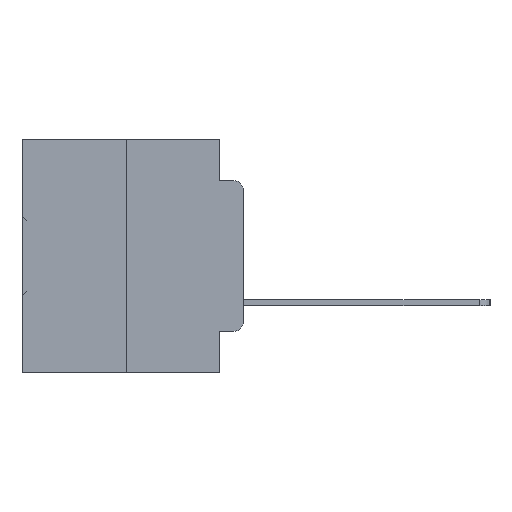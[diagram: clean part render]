
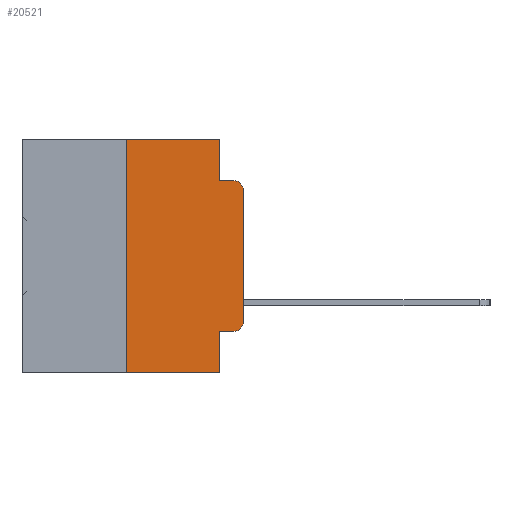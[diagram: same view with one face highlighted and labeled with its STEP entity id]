
A CAD part, left-side view. The second image highlights one B-rep face of the part: STEP entity #20521.
In plain terms, the highlighted planar face has unit normal (-1, 0, 0).
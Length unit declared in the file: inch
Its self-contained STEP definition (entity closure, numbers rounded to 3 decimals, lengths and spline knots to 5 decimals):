
#121 = LINE ( 'NONE', #28309, #34793 ) ;
#863 = DIRECTION ( 'NONE',  ( 0., -1., 0. ) ) ;
#1040 = CARTESIAN_POINT ( 'NONE',  ( 0., 0.25, 0. ) ) ;
#1068 = EDGE_CURVE ( 'NONE', #30678, #3644, #24633, .T. ) ;
#1377 = LINE ( 'NONE', #2020, #29755 ) ;
#2020 = CARTESIAN_POINT ( 'NONE',  ( 0., 0., 0. ) ) ;
#2580 = DIRECTION ( 'NONE',  ( 0., 0., -1. ) ) ;
#2614 = ORIENTED_EDGE ( 'NONE', *, *, #24018, .T. ) ;
#3579 = EDGE_LOOP ( 'NONE', ( #2614, #17501, #33373, #5268, #35038, #14469, #24235, #17936, #12300, #13171 ) ) ;
#3644 = VERTEX_POINT ( 'NONE', #8890 ) ;
#4977 = VERTEX_POINT ( 'NONE', #33874 ) ;
#5185 = AXIS2_PLACEMENT_3D ( 'NONE', #15831, #15921, #26658 ) ;
#5268 = ORIENTED_EDGE ( 'NONE', *, *, #10528, .F. ) ;
#6184 = VECTOR ( 'NONE', #16336, 39.37008 ) ;
#6233 = VECTOR ( 'NONE', #27719, 39.37008 ) ;
#6296 = CARTESIAN_POINT ( 'NONE',  ( 0., 0.051, -0.5 ) ) ;
#6386 = VERTEX_POINT ( 'NONE', #21506 ) ;
#6576 = CARTESIAN_POINT ( 'NONE',  ( 0., 0.051, -0.0885 ) ) ;
#6623 = LINE ( 'NONE', #24682, #20484 ) ;
#8890 = CARTESIAN_POINT ( 'NONE',  ( 0., 0.02, -0.0885 ) ) ;
#10528 = EDGE_CURVE ( 'NONE', #23998, #34937, #26033, .T. ) ;
#11148 = CARTESIAN_POINT ( 'NONE',  ( 0., 0.051, -0.0885 ) ) ;
#11433 = VERTEX_POINT ( 'NONE', #6296 ) ;
#11671 = EDGE_CURVE ( 'NONE', #6386, #18275, #14549, .T. ) ;
#12300 = ORIENTED_EDGE ( 'NONE', *, *, #12589, .T. ) ;
#12589 = EDGE_CURVE ( 'NONE', #4977, #23850, #22583, .T. ) ;
#12897 = CARTESIAN_POINT ( 'NONE',  ( 0., 0.02, -0.3915 ) ) ;
#13171 = ORIENTED_EDGE ( 'NONE', *, *, #20290, .T. ) ;
#13213 = CARTESIAN_POINT ( 'NONE',  ( 0., 0.051, 0. ) ) ;
#13529 = CARTESIAN_POINT ( 'NONE',  ( 0., 0.051, -0.4115 ) ) ;
#13761 = PLANE ( 'NONE',  #28790 ) ;
#14206 = VECTOR ( 'NONE', #863, 39.37008 ) ;
#14469 = ORIENTED_EDGE ( 'NONE', *, *, #11671, .F. ) ;
#14549 = LINE ( 'NONE', #1040, #35109 ) ;
#14850 = DIRECTION ( 'NONE',  ( 0., 0., -1. ) ) ;
#15708 = DIRECTION ( 'NONE',  ( 0., 0., -1. ) ) ;
#15831 = CARTESIAN_POINT ( 'NONE',  ( 0., 0.02, -0.1085 ) ) ;
#15921 = DIRECTION ( 'NONE',  ( -1., 0., 0. ) ) ;
#16018 = DIRECTION ( 'NONE',  ( 0., 0., -1. ) ) ;
#16134 = EDGE_CURVE ( 'NONE', #34937, #3644, #28594, .T. ) ;
#16336 = DIRECTION ( 'NONE',  ( 0., -1., 0. ) ) ;
#17501 = ORIENTED_EDGE ( 'NONE', *, *, #1068, .T. ) ;
#17936 = ORIENTED_EDGE ( 'NONE', *, *, #33659, .F. ) ;
#18275 = VERTEX_POINT ( 'NONE', #27821 ) ;
#18853 = FACE_OUTER_BOUND ( 'NONE', #3579, .T. ) ;
#19296 = DIRECTION ( 'NONE',  ( 1., 0., 0. ) ) ;
#20290 = EDGE_CURVE ( 'NONE', #23850, #25393, #32629, .T. ) ;
#20484 = VECTOR ( 'NONE', #27399, 39.37008 ) ;
#20521 = ADVANCED_FACE ( 'NONE', ( #18853 ), #13761, .F. ) ;
#20655 = EDGE_CURVE ( 'NONE', #6386, #11433, #20956, .T. ) ;
#20956 = LINE ( 'NONE', #22330, #6233 ) ;
#21506 = CARTESIAN_POINT ( 'NONE',  ( 0., 0.25, -0.5 ) ) ;
#21876 = CARTESIAN_POINT ( 'NONE',  ( 0., 0.473, 0. ) ) ;
#22330 = CARTESIAN_POINT ( 'NONE',  ( 0., 0.473, -0.5 ) ) ;
#22583 = LINE ( 'NONE', #13529, #6184 ) ;
#23850 = VERTEX_POINT ( 'NONE', #31482 ) ;
#23998 = VERTEX_POINT ( 'NONE', #26866 ) ;
#24018 = EDGE_CURVE ( 'NONE', #25393, #30678, #1377, .T. ) ;
#24235 = ORIENTED_EDGE ( 'NONE', *, *, #20655, .T. ) ;
#24633 = CIRCLE ( 'NONE', #5185, 0.02 ) ;
#24682 = CARTESIAN_POINT ( 'NONE',  ( 0., 0.473, 0. ) ) ;
#25393 = VERTEX_POINT ( 'NONE', #33356 ) ;
#26033 = LINE ( 'NONE', #13213, #31427 ) ;
#26658 = DIRECTION ( 'NONE',  ( 0., 0., -1. ) ) ;
#26866 = CARTESIAN_POINT ( 'NONE',  ( 0., 0.051, 0. ) ) ;
#26977 = DIRECTION ( 'NONE',  ( 0., 0., 1. ) ) ;
#27399 = DIRECTION ( 'NONE',  ( 0., -1., 0. ) ) ;
#27719 = DIRECTION ( 'NONE',  ( 0., -1., 0. ) ) ;
#27821 = CARTESIAN_POINT ( 'NONE',  ( 0., 0.25, 0. ) ) ;
#28309 = CARTESIAN_POINT ( 'NONE',  ( 0., 0.051, 0. ) ) ;
#28594 = LINE ( 'NONE', #6576, #14206 ) ;
#28790 = AXIS2_PLACEMENT_3D ( 'NONE', #21876, #19296, #2580 ) ;
#29755 = VECTOR ( 'NONE', #26977, 39.37008 ) ;
#29921 = CARTESIAN_POINT ( 'NONE',  ( 0., 0., -0.1085 ) ) ;
#30678 = VERTEX_POINT ( 'NONE', #29921 ) ;
#31427 = VECTOR ( 'NONE', #16018, 39.37008 ) ;
#31482 = CARTESIAN_POINT ( 'NONE',  ( 0., 0.02, -0.4115 ) ) ;
#31777 = DIRECTION ( 'NONE',  ( -1., 0., 0. ) ) ;
#32629 = CIRCLE ( 'NONE', #32965, 0.02 ) ;
#32965 = AXIS2_PLACEMENT_3D ( 'NONE', #12897, #31777, #15708 ) ;
#33356 = CARTESIAN_POINT ( 'NONE',  ( 0., 0., -0.3915 ) ) ;
#33373 = ORIENTED_EDGE ( 'NONE', *, *, #16134, .F. ) ;
#33659 = EDGE_CURVE ( 'NONE', #4977, #11433, #121, .T. ) ;
#33809 = DIRECTION ( 'NONE',  ( 0., 0., 1. ) ) ;
#33874 = CARTESIAN_POINT ( 'NONE',  ( 0., 0.051, -0.4115 ) ) ;
#34257 = EDGE_CURVE ( 'NONE', #18275, #23998, #6623, .T. ) ;
#34793 = VECTOR ( 'NONE', #14850, 39.37008 ) ;
#34937 = VERTEX_POINT ( 'NONE', #11148 ) ;
#35038 = ORIENTED_EDGE ( 'NONE', *, *, #34257, .F. ) ;
#35109 = VECTOR ( 'NONE', #33809, 39.37008 ) ;
